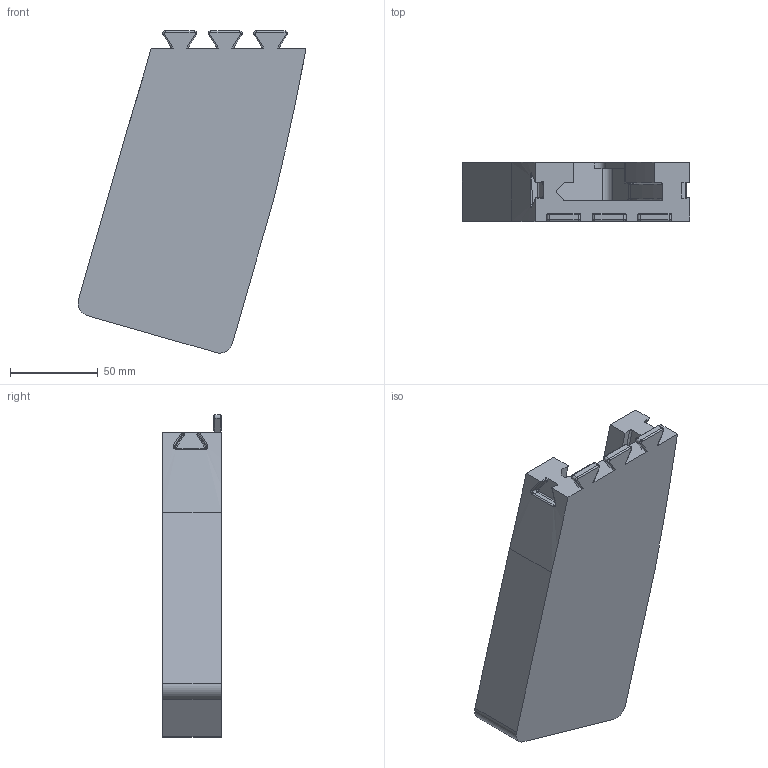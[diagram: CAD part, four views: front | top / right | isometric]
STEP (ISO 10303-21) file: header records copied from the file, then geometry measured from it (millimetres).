
FILE_DESCRIPTION(/* description */ (''),/* implementation_level */ '2;1');
FILE_NAME(/* name */ 'freeman1337_ar15-mag-speedloader-tray-v5.step',/* time_stamp */ '2021-09-04T08:15:57-07:00',/* author */ (''),/* organization */ (''),/* preprocessor_version */ 'ST-DEVELOPER v18.1',/* originating_system */ 'Autodesk Translation Framework v10.10.0.1391',/* authorisation */ '');
FILE_SCHEMA (('AUTOMOTIVE_DESIGN { 1 0 10303 214 3 1 1 }'));
Length unit declared in the file: millimetre
Products named in the file (1): loader-tray
Bounding box: 129.97 x 33.62 x 183.66 mm (x, y, z)
Volume: 275896 mm3; surface area: 59773.9 mm2
Topology: 1 solids, 1 shells, 151 faces, 392 edges, 242 vertices
Faces by surface type: cylinder 63, plane 47, bspline 41
Entity records: 5419 total; most frequent: CARTESIAN_POINT 1784, ORIENTED_EDGE 782, DIRECTION 751, EDGE_CURVE 391, AXIS2_PLACEMENT_3D 283, VERTEX_POINT 242, LINE 185, VECTOR 185
